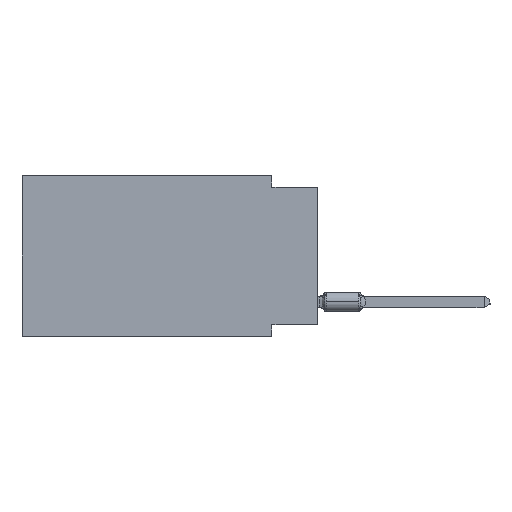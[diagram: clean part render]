
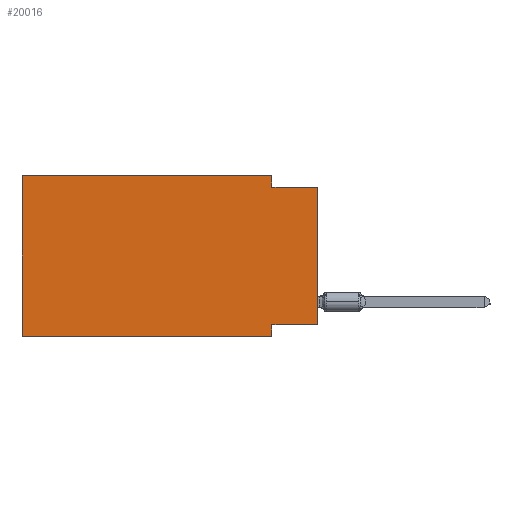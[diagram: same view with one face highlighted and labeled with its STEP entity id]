
A CAD part, left-side view. The second image highlights one B-rep face of the part: STEP entity #20016.
In plain terms, the highlighted planar face has unit normal (-1, 0, 0).
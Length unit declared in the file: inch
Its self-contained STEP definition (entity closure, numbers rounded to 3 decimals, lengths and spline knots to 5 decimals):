
#103 = LINE ( 'NONE', #1504, #6705 ) ;
#136 = DIRECTION ( 'NONE',  ( 1., 0., 0. ) ) ;
#1117 = FACE_OUTER_BOUND ( 'NONE', #14328, .T. ) ;
#1379 = CARTESIAN_POINT ( 'NONE',  ( 0., 0., -0.025 ) ) ;
#1504 = CARTESIAN_POINT ( 'NONE',  ( 0., 0.645, 0. ) ) ;
#1836 = VECTOR ( 'NONE', #10577, 39.37008 ) ;
#1853 = DIRECTION ( 'NONE',  ( 0., 0., -1. ) ) ;
#2225 = CARTESIAN_POINT ( 'NONE',  ( 0., 0.645, 0. ) ) ;
#2580 = CARTESIAN_POINT ( 'NONE',  ( 0., 0.1, -0.025 ) ) ;
#2832 = PLANE ( 'NONE',  #17233 ) ;
#3060 = ORIENTED_EDGE ( 'NONE', *, *, #18178, .F. ) ;
#3131 = VERTEX_POINT ( 'NONE', #9660 ) ;
#3783 = ORIENTED_EDGE ( 'NONE', *, *, #12894, .F. ) ;
#4243 = LINE ( 'NONE', #10784, #14763 ) ;
#4528 = VERTEX_POINT ( 'NONE', #2580 ) ;
#4989 = LINE ( 'NONE', #14741, #10015 ) ;
#5169 = CARTESIAN_POINT ( 'NONE',  ( 0., 0.645, 0. ) ) ;
#5984 = EDGE_CURVE ( 'NONE', #14606, #10133, #103, .T. ) ;
#6081 = LINE ( 'NONE', #19287, #8252 ) ;
#6357 = DIRECTION ( 'NONE',  ( 0., 0., -1. ) ) ;
#6705 = VECTOR ( 'NONE', #8040, 39.37008 ) ;
#7695 = CARTESIAN_POINT ( 'NONE',  ( 0., 0., -0.325 ) ) ;
#8040 = DIRECTION ( 'NONE',  ( 0., -1., 0. ) ) ;
#8252 = VECTOR ( 'NONE', #9617, 39.37008 ) ;
#9617 = DIRECTION ( 'NONE',  ( 0., 1., 0. ) ) ;
#9660 = CARTESIAN_POINT ( 'NONE',  ( 0., 0.645, -0.35 ) ) ;
#9857 = EDGE_CURVE ( 'NONE', #16043, #19275, #19349, .T. ) ;
#9901 = EDGE_CURVE ( 'NONE', #16809, #18684, #21061, .T. ) ;
#10015 = VECTOR ( 'NONE', #15163, 39.37008 ) ;
#10111 = CARTESIAN_POINT ( 'NONE',  ( 0., 0.1, -0.325 ) ) ;
#10133 = VERTEX_POINT ( 'NONE', #20484 ) ;
#10577 = DIRECTION ( 'NONE',  ( 0., 0., 1. ) ) ;
#10784 = CARTESIAN_POINT ( 'NONE',  ( 0., 0., -0.025 ) ) ;
#11084 = CARTESIAN_POINT ( 'NONE',  ( 0., 0.1, -0.35 ) ) ;
#11232 = VECTOR ( 'NONE', #16336, 39.37008 ) ;
#12222 = DIRECTION ( 'NONE',  ( 0., 0., -1. ) ) ;
#12242 = VECTOR ( 'NONE', #6357, 39.37008 ) ;
#12894 = EDGE_CURVE ( 'NONE', #10133, #4528, #13830, .T. ) ;
#13164 = CARTESIAN_POINT ( 'NONE',  ( 0., 0.645, 0. ) ) ;
#13345 = ORIENTED_EDGE ( 'NONE', *, *, #13399, .F. ) ;
#13399 = EDGE_CURVE ( 'NONE', #16043, #16809, #6081, .T. ) ;
#13830 = LINE ( 'NONE', #20381, #19544 ) ;
#13893 = LINE ( 'NONE', #2225, #1836 ) ;
#14328 = EDGE_LOOP ( 'NONE', ( #15818, #14552, #3783, #17082, #3060, #18228, #14504, #13345 ) ) ;
#14409 = CARTESIAN_POINT ( 'NONE',  ( 0., 0., 0. ) ) ;
#14504 = ORIENTED_EDGE ( 'NONE', *, *, #9901, .F. ) ;
#14552 = ORIENTED_EDGE ( 'NONE', *, *, #15327, .F. ) ;
#14606 = VERTEX_POINT ( 'NONE', #13164 ) ;
#14741 = CARTESIAN_POINT ( 'NONE',  ( 0., 0.645, -0.35 ) ) ;
#14763 = VECTOR ( 'NONE', #17332, 39.37008 ) ;
#15163 = DIRECTION ( 'NONE',  ( 0., -1., 0. ) ) ;
#15327 = EDGE_CURVE ( 'NONE', #4528, #19275, #4243, .T. ) ;
#15818 = ORIENTED_EDGE ( 'NONE', *, *, #9857, .T. ) ;
#16043 = VERTEX_POINT ( 'NONE', #7695 ) ;
#16336 = DIRECTION ( 'NONE',  ( 0., 0., 1. ) ) ;
#16809 = VERTEX_POINT ( 'NONE', #10111 ) ;
#17082 = ORIENTED_EDGE ( 'NONE', *, *, #5984, .F. ) ;
#17233 = AXIS2_PLACEMENT_3D ( 'NONE', #5169, #136, #1853 ) ;
#17332 = DIRECTION ( 'NONE',  ( 0., -1., 0. ) ) ;
#18178 = EDGE_CURVE ( 'NONE', #3131, #14606, #13893, .T. ) ;
#18228 = ORIENTED_EDGE ( 'NONE', *, *, #19719, .T. ) ;
#18684 = VERTEX_POINT ( 'NONE', #18708 ) ;
#18708 = CARTESIAN_POINT ( 'NONE',  ( 0., 0.1, -0.35 ) ) ;
#19275 = VERTEX_POINT ( 'NONE', #1379 ) ;
#19287 = CARTESIAN_POINT ( 'NONE',  ( 0., 0., -0.325 ) ) ;
#19349 = LINE ( 'NONE', #14409, #11232 ) ;
#19544 = VECTOR ( 'NONE', #12222, 39.37008 ) ;
#19719 = EDGE_CURVE ( 'NONE', #3131, #18684, #4989, .T. ) ;
#20016 = ADVANCED_FACE ( 'NONE', ( #1117 ), #2832, .F. ) ;
#20381 = CARTESIAN_POINT ( 'NONE',  ( 0., 0.1, 0. ) ) ;
#20484 = CARTESIAN_POINT ( 'NONE',  ( 0., 0.1, 0. ) ) ;
#21061 = LINE ( 'NONE', #11084, #12242 ) ;
